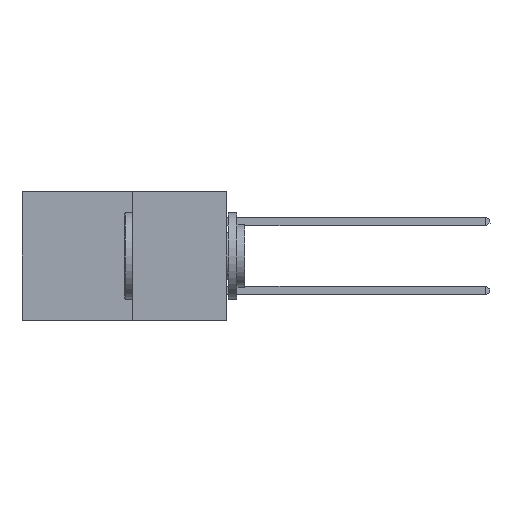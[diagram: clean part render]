
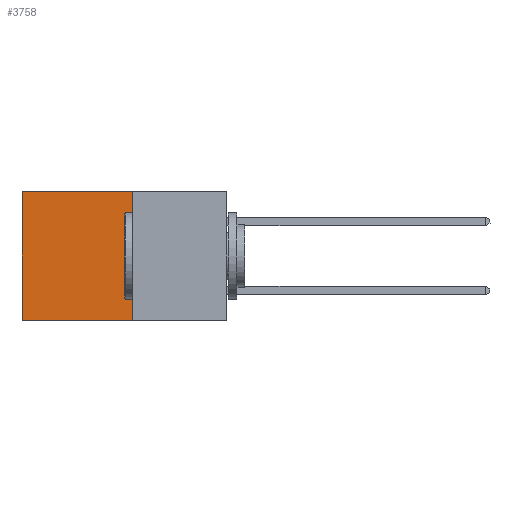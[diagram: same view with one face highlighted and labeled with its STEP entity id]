
A CAD part, left-side view. The second image highlights one B-rep face of the part: STEP entity #3758.
In plain terms, the highlighted planar face has unit normal (-1, 0, 0).
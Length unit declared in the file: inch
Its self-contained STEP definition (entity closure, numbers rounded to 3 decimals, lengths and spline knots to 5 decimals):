
#102 = ORIENTED_EDGE ( 'NONE', *, *, #763, .T. ) ;
#638 = VECTOR ( 'NONE', #6360, 39.37008 ) ;
#763 = EDGE_CURVE ( 'NONE', #1225, #1545, #8448, .T. ) ;
#1109 = VERTEX_POINT ( 'NONE', #7526 ) ;
#1225 = VERTEX_POINT ( 'NONE', #5233 ) ;
#1545 = VERTEX_POINT ( 'NONE', #4017 ) ;
#1841 = CARTESIAN_POINT ( 'NONE',  ( 0.277, 0.27, 0. ) ) ;
#1993 = VERTEX_POINT ( 'NONE', #1841 ) ;
#2117 = FACE_OUTER_BOUND ( 'NONE', #7161, .T. ) ;
#2513 = LINE ( 'NONE', #3767, #4180 ) ;
#2590 = CARTESIAN_POINT ( 'NONE',  ( 0.277, 0.27, 0. ) ) ;
#2634 = ORIENTED_EDGE ( 'NONE', *, *, #7577, .F. ) ;
#2668 = LINE ( 'NONE', #6552, #638 ) ;
#3361 = ORIENTED_EDGE ( 'NONE', *, *, #4928, .F. ) ;
#3758 = ADVANCED_FACE ( 'NONE', ( #2117 ), #6786, .F. ) ;
#3767 = CARTESIAN_POINT ( 'NONE',  ( 0.277, 0.27, -0.37 ) ) ;
#4017 = CARTESIAN_POINT ( 'NONE',  ( 0.277, 0.59, -0.37 ) ) ;
#4180 = VECTOR ( 'NONE', #4530, 39.37008 ) ;
#4451 = VECTOR ( 'NONE', #6390, 39.37008 ) ;
#4530 = DIRECTION ( 'NONE',  ( 0., 0., -1. ) ) ;
#4746 = AXIS2_PLACEMENT_3D ( 'NONE', #5035, #7940, #7609 ) ;
#4888 = LINE ( 'NONE', #2590, #6410 ) ;
#4928 = EDGE_CURVE ( 'NONE', #1109, #1545, #2668, .T. ) ;
#5035 = CARTESIAN_POINT ( 'NONE',  ( 0.277, 0.27, -0.37 ) ) ;
#5233 = CARTESIAN_POINT ( 'NONE',  ( 0.277, 0.59, 0. ) ) ;
#6058 = DIRECTION ( 'NONE',  ( 0., 1., 0. ) ) ;
#6360 = DIRECTION ( 'NONE',  ( 0., 1., 0. ) ) ;
#6390 = DIRECTION ( 'NONE',  ( 0., 0., -1. ) ) ;
#6410 = VECTOR ( 'NONE', #6058, 39.37008 ) ;
#6520 = CARTESIAN_POINT ( 'NONE',  ( 0.277, 0.59, -0.37 ) ) ;
#6552 = CARTESIAN_POINT ( 'NONE',  ( 0.277, 0.27, -0.37 ) ) ;
#6786 = PLANE ( 'NONE',  #4746 ) ;
#6912 = ORIENTED_EDGE ( 'NONE', *, *, #7012, .T. ) ;
#7012 = EDGE_CURVE ( 'NONE', #1993, #1225, #4888, .T. ) ;
#7161 = EDGE_LOOP ( 'NONE', ( #102, #3361, #2634, #6912 ) ) ;
#7526 = CARTESIAN_POINT ( 'NONE',  ( 0.277, 0.27, -0.37 ) ) ;
#7577 = EDGE_CURVE ( 'NONE', #1993, #1109, #2513, .T. ) ;
#7609 = DIRECTION ( 'NONE',  ( 0., 0., -1. ) ) ;
#7940 = DIRECTION ( 'NONE',  ( 1., 0., 0. ) ) ;
#8448 = LINE ( 'NONE', #6520, #4451 ) ;
